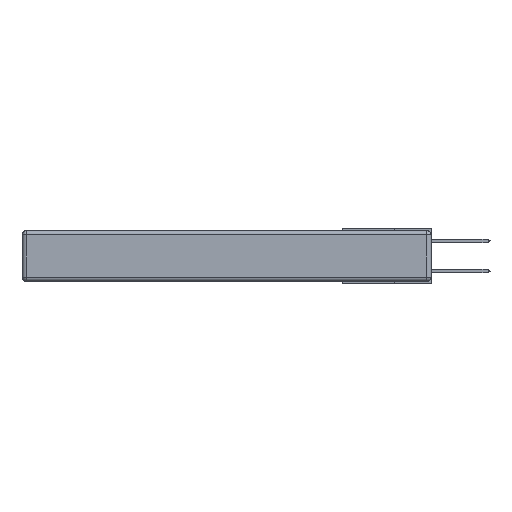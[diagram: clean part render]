
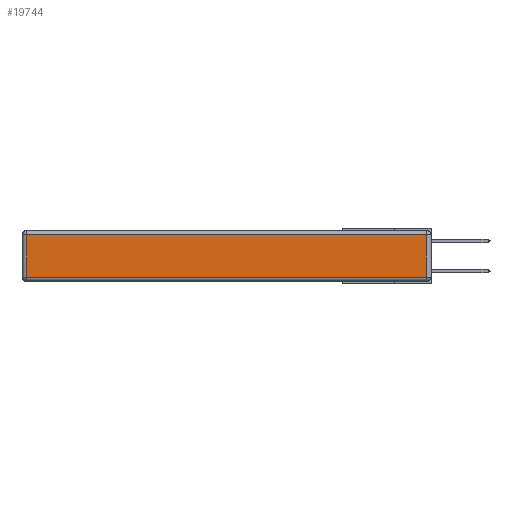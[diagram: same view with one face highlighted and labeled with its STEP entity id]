
A CAD part, left-side view. The second image highlights one B-rep face of the part: STEP entity #19744.
In plain terms, the highlighted planar face has unit normal (-1, 0, 0).
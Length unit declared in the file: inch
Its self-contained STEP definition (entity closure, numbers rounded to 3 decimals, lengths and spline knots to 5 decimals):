
#298 = VERTEX_POINT ( 'NONE', #4970 ) ;
#654 = CARTESIAN_POINT ( 'NONE',  ( 0., 0.03, -0.343 ) ) ;
#1648 = EDGE_LOOP ( 'NONE', ( #28154, #20914, #9331, #32774 ) ) ;
#2951 = DIRECTION ( 'NONE',  ( 0., 1., 0. ) ) ;
#3402 = VERTEX_POINT ( 'NONE', #8158 ) ;
#3415 = EDGE_CURVE ( 'NONE', #3402, #298, #3573, .T. ) ;
#3573 = LINE ( 'NONE', #654, #20143 ) ;
#4058 = EDGE_CURVE ( 'NONE', #23052, #3402, #20878, .T. ) ;
#4687 = CARTESIAN_POINT ( 'NONE',  ( 0., 2.75, -0.03 ) ) ;
#4970 = CARTESIAN_POINT ( 'NONE',  ( 0., 0.03, -0.03 ) ) ;
#5642 = VERTEX_POINT ( 'NONE', #12821 ) ;
#5873 = DIRECTION ( 'NONE',  ( 0., 0., 1. ) ) ;
#6757 = VECTOR ( 'NONE', #14346, 39.37008 ) ;
#8158 = CARTESIAN_POINT ( 'NONE',  ( 0., 0.03, -0.313 ) ) ;
#8263 = VECTOR ( 'NONE', #2951, 39.37008 ) ;
#8370 = LINE ( 'NONE', #32564, #6757 ) ;
#9331 = ORIENTED_EDGE ( 'NONE', *, *, #21170, .T. ) ;
#12821 = CARTESIAN_POINT ( 'NONE',  ( 0., 2.72, -0.03 ) ) ;
#14164 = DIRECTION ( 'NONE',  ( -1., 0., 0. ) ) ;
#14346 = DIRECTION ( 'NONE',  ( 0., 0., -1. ) ) ;
#16736 = LINE ( 'NONE', #4687, #8263 ) ;
#18880 = VECTOR ( 'NONE', #28984, 39.37008 ) ;
#18991 = CARTESIAN_POINT ( 'NONE',  ( 0., 0., -0.313 ) ) ;
#19690 = AXIS2_PLACEMENT_3D ( 'NONE', #26724, #14164, #32164 ) ;
#19744 = ADVANCED_FACE ( 'NONE', ( #33347 ), #24137, .T. ) ;
#20143 = VECTOR ( 'NONE', #5873, 39.37008 ) ;
#20878 = LINE ( 'NONE', #18991, #18880 ) ;
#20914 = ORIENTED_EDGE ( 'NONE', *, *, #3415, .T. ) ;
#21170 = EDGE_CURVE ( 'NONE', #298, #5642, #16736, .T. ) ;
#23052 = VERTEX_POINT ( 'NONE', #30515 ) ;
#24137 = PLANE ( 'NONE',  #19690 ) ;
#26724 = CARTESIAN_POINT ( 'NONE',  ( 0., 0., -0.343 ) ) ;
#28154 = ORIENTED_EDGE ( 'NONE', *, *, #4058, .T. ) ;
#28984 = DIRECTION ( 'NONE',  ( 0., -1., 0. ) ) ;
#30515 = CARTESIAN_POINT ( 'NONE',  ( 0., 2.72, -0.313 ) ) ;
#32164 = DIRECTION ( 'NONE',  ( 0., 0., 1. ) ) ;
#32456 = EDGE_CURVE ( 'NONE', #5642, #23052, #8370, .T. ) ;
#32564 = CARTESIAN_POINT ( 'NONE',  ( 0., 2.72, -0.343 ) ) ;
#32774 = ORIENTED_EDGE ( 'NONE', *, *, #32456, .T. ) ;
#33347 = FACE_OUTER_BOUND ( 'NONE', #1648, .T. ) ;
